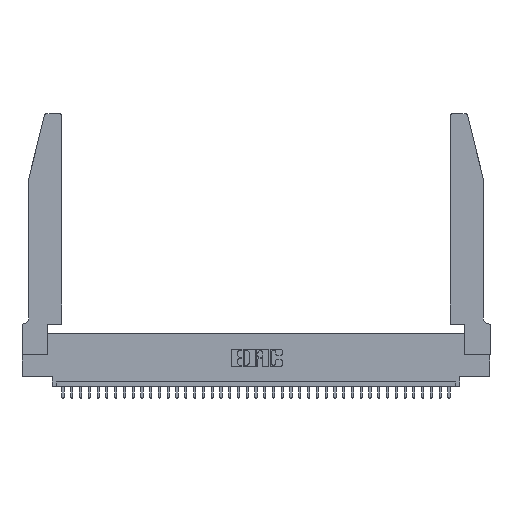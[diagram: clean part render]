
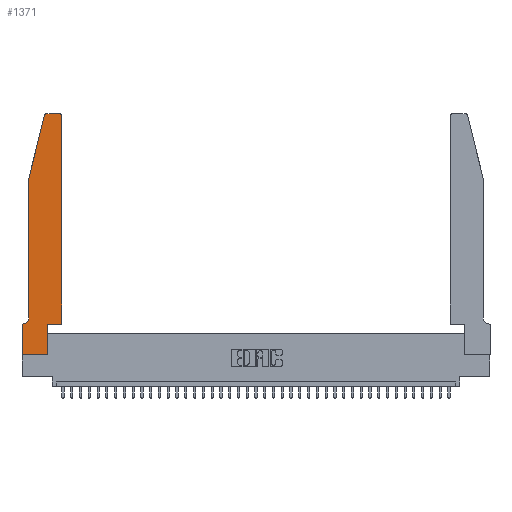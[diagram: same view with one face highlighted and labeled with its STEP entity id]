
A CAD part, top view. The second image highlights one B-rep face of the part: STEP entity #1371.
In plain terms, the highlighted planar face has unit normal (0, 0, 1).
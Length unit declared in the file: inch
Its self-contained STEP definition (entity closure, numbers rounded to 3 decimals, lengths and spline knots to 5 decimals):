
#294 = LINE ( 'NONE', #19122, #23943 ) ;
#1198 = DIRECTION ( 'NONE',  ( 0., 1., 0. ) ) ;
#1371 = ADVANCED_FACE ( 'NONE', ( #37096 ), #28638, .T. ) ;
#1538 = ORIENTED_EDGE ( 'NONE', *, *, #31989, .T. ) ;
#1711 = LINE ( 'NONE', #18647, #21127 ) ;
#2304 = VERTEX_POINT ( 'NONE', #19690 ) ;
#2647 = CARTESIAN_POINT ( 'NONE',  ( 0.4505, 0.35, 0.37 ) ) ;
#2826 = CARTESIAN_POINT ( 'NONE',  ( 0.0755, 0.35, 0.37 ) ) ;
#2913 = AXIS2_PLACEMENT_3D ( 'NONE', #13437, #25634, #37418 ) ;
#2961 = VECTOR ( 'NONE', #21200, 39.37008 ) ;
#3447 = CARTESIAN_POINT ( 'NONE',  ( 0.0755, 2., 0.37 ) ) ;
#3593 = AXIS2_PLACEMENT_3D ( 'NONE', #9279, #30380, #6421 ) ;
#3939 = VECTOR ( 'NONE', #6396, 39.37008 ) ;
#4045 = CARTESIAN_POINT ( 'NONE',  ( 0.284, 2.75, 0.37 ) ) ;
#4165 = VERTEX_POINT ( 'NONE', #16230 ) ;
#4302 = LINE ( 'NONE', #6053, #2961 ) ;
#4614 = CARTESIAN_POINT ( 'NONE',  ( 0.4205, 2.72, 0.37 ) ) ;
#5539 = VERTEX_POINT ( 'NONE', #33585 ) ;
#5693 = EDGE_CURVE ( 'NONE', #28039, #5539, #34020, .T. ) ;
#6053 = CARTESIAN_POINT ( 'NONE',  ( 0., 0., 0.37 ) ) ;
#6208 = VECTOR ( 'NONE', #21919, 39.37008 ) ;
#6396 = DIRECTION ( 'NONE',  ( 0., -1., 0. ) ) ;
#6421 = DIRECTION ( 'NONE',  ( 1., 0., 0. ) ) ;
#6752 = LINE ( 'NONE', #24141, #14666 ) ;
#7118 = CARTESIAN_POINT ( 'NONE',  ( 0.4505, 0.35, 0.37 ) ) ;
#7760 = EDGE_CURVE ( 'NONE', #30047, #4165, #10215, .T. ) ;
#7773 = AXIS2_PLACEMENT_3D ( 'NONE', #23962, #20726, #9045 ) ;
#8227 = ORIENTED_EDGE ( 'NONE', *, *, #19643, .T. ) ;
#8401 = CIRCLE ( 'NONE', #26597, 0.03 ) ;
#8542 = ORIENTED_EDGE ( 'NONE', *, *, #18617, .T. ) ;
#9045 = DIRECTION ( 'NONE',  ( -1., 0., 0. ) ) ;
#9279 = CARTESIAN_POINT ( 'NONE',  ( 0.284, 2.72, 0.37 ) ) ;
#9705 = VERTEX_POINT ( 'NONE', #14139 ) ;
#10215 = LINE ( 'NONE', #2826, #15279 ) ;
#11710 = DIRECTION ( 'NONE',  ( -1., 0., 0. ) ) ;
#11795 = DIRECTION ( 'NONE',  ( 1., 0., 0. ) ) ;
#11813 = LINE ( 'NONE', #3447, #3939 ) ;
#12281 = CARTESIAN_POINT ( 'NONE',  ( 0.2605, 2.75, 0.37 ) ) ;
#12635 = VERTEX_POINT ( 'NONE', #17151 ) ;
#13437 = CARTESIAN_POINT ( 'NONE',  ( 0., 0.35, 0.37 ) ) ;
#14139 = CARTESIAN_POINT ( 'NONE',  ( 0.0755, 0.42, 0.37 ) ) ;
#14666 = VECTOR ( 'NONE', #15729, 39.37008 ) ;
#14914 = CARTESIAN_POINT ( 'NONE',  ( 0.0055, 0.35, 0.37 ) ) ;
#15279 = VECTOR ( 'NONE', #11710, 39.37008 ) ;
#15729 = DIRECTION ( 'NONE',  ( 0., 1., 0. ) ) ;
#16155 = DIRECTION ( 'NONE',  ( 1., 0., 0. ) ) ;
#16230 = CARTESIAN_POINT ( 'NONE',  ( 0., 0.35, 0.37 ) ) ;
#16307 = VERTEX_POINT ( 'NONE', #19267 ) ;
#17119 = CARTESIAN_POINT ( 'NONE',  ( 0.2865, 0., 0.37 ) ) ;
#17151 = CARTESIAN_POINT ( 'NONE',  ( 0.4205, 2.75, 0.37 ) ) ;
#17368 = VERTEX_POINT ( 'NONE', #4045 ) ;
#17875 = EDGE_CURVE ( 'NONE', #9705, #30047, #24970, .T. ) ;
#18385 = VECTOR ( 'NONE', #11795, 39.37008 ) ;
#18476 = EDGE_CURVE ( 'NONE', #4165, #16307, #294, .T. ) ;
#18535 = ORIENTED_EDGE ( 'NONE', *, *, #23833, .T. ) ;
#18617 = EDGE_CURVE ( 'NONE', #21837, #28039, #34228, .T. ) ;
#18647 = CARTESIAN_POINT ( 'NONE',  ( 0.0755, 2., 0.37 ) ) ;
#18745 = EDGE_CURVE ( 'NONE', #27410, #2304, #1711, .T. ) ;
#19122 = CARTESIAN_POINT ( 'NONE',  ( 0., 0., 0.37 ) ) ;
#19267 = CARTESIAN_POINT ( 'NONE',  ( 0., 0., 0.37 ) ) ;
#19537 = DIRECTION ( 'NONE',  ( 0., 0., 1. ) ) ;
#19643 = EDGE_CURVE ( 'NONE', #2304, #9705, #11813, .T. ) ;
#19690 = CARTESIAN_POINT ( 'NONE',  ( 0.0755, 2., 0.37 ) ) ;
#20293 = ORIENTED_EDGE ( 'NONE', *, *, #28804, .T. ) ;
#20726 = DIRECTION ( 'NONE',  ( 0., 0., -1. ) ) ;
#21127 = VECTOR ( 'NONE', #35753, 39.37008 ) ;
#21200 = DIRECTION ( 'NONE',  ( 1., 0., 0. ) ) ;
#21837 = VERTEX_POINT ( 'NONE', #28960 ) ;
#21919 = DIRECTION ( 'NONE',  ( -1., 0., 0. ) ) ;
#22978 = EDGE_LOOP ( 'NONE', ( #18535, #28466, #30900, #8227, #27003, #32575, #25110, #20293, #1538, #8542, #34310, #25363 ) ) ;
#23481 = CIRCLE ( 'NONE', #3593, 0.03 ) ;
#23833 = EDGE_CURVE ( 'NONE', #12635, #17368, #37801, .T. ) ;
#23943 = VECTOR ( 'NONE', #28068, 39.37008 ) ;
#23962 = CARTESIAN_POINT ( 'NONE',  ( 0.0055, 0.42, 0.37 ) ) ;
#24141 = CARTESIAN_POINT ( 'NONE',  ( 0.2865, 0.35, 0.37 ) ) ;
#24426 = CARTESIAN_POINT ( 'NONE',  ( 0.4505, 0.35, 0.37 ) ) ;
#24970 = CIRCLE ( 'NONE', #7773, 0.07 ) ;
#25110 = ORIENTED_EDGE ( 'NONE', *, *, #18476, .T. ) ;
#25363 = ORIENTED_EDGE ( 'NONE', *, *, #25902, .T. ) ;
#25634 = DIRECTION ( 'NONE',  ( 0., 0., 1. ) ) ;
#25902 = EDGE_CURVE ( 'NONE', #5539, #12635, #8401, .T. ) ;
#26597 = AXIS2_PLACEMENT_3D ( 'NONE', #4614, #19537, #16155 ) ;
#26751 = VERTEX_POINT ( 'NONE', #17119 ) ;
#27003 = ORIENTED_EDGE ( 'NONE', *, *, #17875, .T. ) ;
#27410 = VERTEX_POINT ( 'NONE', #29164 ) ;
#28039 = VERTEX_POINT ( 'NONE', #24426 ) ;
#28068 = DIRECTION ( 'NONE',  ( 0., -1., 0. ) ) ;
#28466 = ORIENTED_EDGE ( 'NONE', *, *, #33351, .T. ) ;
#28638 = PLANE ( 'NONE',  #2913 ) ;
#28804 = EDGE_CURVE ( 'NONE', #16307, #26751, #4302, .T. ) ;
#28922 = VECTOR ( 'NONE', #1198, 39.37008 ) ;
#28960 = CARTESIAN_POINT ( 'NONE',  ( 0.2865, 0.35, 0.37 ) ) ;
#29164 = CARTESIAN_POINT ( 'NONE',  ( 0.25487, 2.72718, 0.37 ) ) ;
#30047 = VERTEX_POINT ( 'NONE', #14914 ) ;
#30380 = DIRECTION ( 'NONE',  ( 0., 0., 1. ) ) ;
#30900 = ORIENTED_EDGE ( 'NONE', *, *, #18745, .T. ) ;
#31989 = EDGE_CURVE ( 'NONE', #26751, #21837, #6752, .T. ) ;
#32575 = ORIENTED_EDGE ( 'NONE', *, *, #7760, .T. ) ;
#33351 = EDGE_CURVE ( 'NONE', #17368, #27410, #23481, .T. ) ;
#33585 = CARTESIAN_POINT ( 'NONE',  ( 0.4505, 2.72, 0.37 ) ) ;
#34020 = LINE ( 'NONE', #7118, #28922 ) ;
#34228 = LINE ( 'NONE', #2647, #18385 ) ;
#34310 = ORIENTED_EDGE ( 'NONE', *, *, #5693, .T. ) ;
#35753 = DIRECTION ( 'NONE',  ( -0.239, -0.971, 0. ) ) ;
#37096 = FACE_OUTER_BOUND ( 'NONE', #22978, .T. ) ;
#37418 = DIRECTION ( 'NONE',  ( 1., 0., 0. ) ) ;
#37801 = LINE ( 'NONE', #12281, #6208 ) ;
